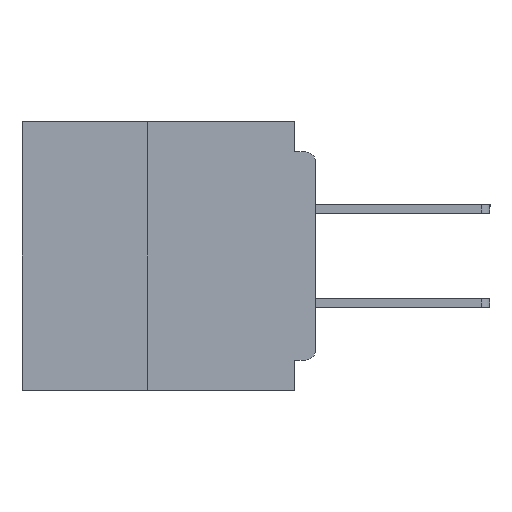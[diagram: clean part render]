
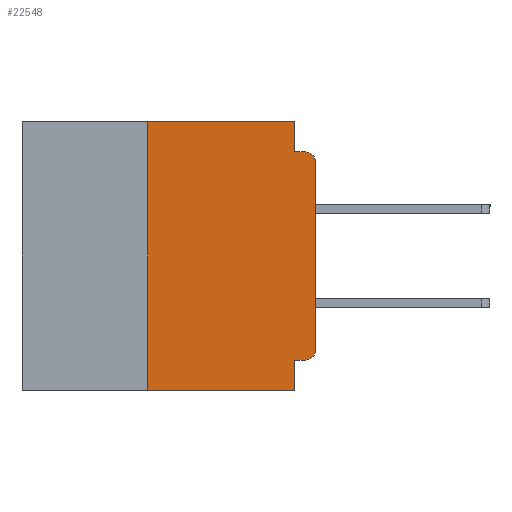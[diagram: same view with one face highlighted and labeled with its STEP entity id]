
A CAD part, left-side view. The second image highlights one B-rep face of the part: STEP entity #22548.
In plain terms, the highlighted planar face has unit normal (-1, 0, 0).
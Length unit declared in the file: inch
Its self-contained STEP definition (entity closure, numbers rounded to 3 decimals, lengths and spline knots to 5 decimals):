
#13 = CARTESIAN_POINT ( 'NONE',  ( 0., 0.25, -0.4 ) ) ;
#24 = VECTOR ( 'NONE', #770, 39.37008 ) ;
#57 = ORIENTED_EDGE ( 'NONE', *, *, #15353, .F. ) ;
#374 = VECTOR ( 'NONE', #3864, 39.37008 ) ;
#440 = EDGE_CURVE ( 'NONE', #1643, #30247, #30503, .T. ) ;
#537 = CARTESIAN_POINT ( 'NONE',  ( 0., 0.031, -0.355 ) ) ;
#770 = DIRECTION ( 'NONE',  ( 0., 0., -1. ) ) ;
#933 = PLANE ( 'NONE',  #33483 ) ;
#1409 = VECTOR ( 'NONE', #37729, 39.37008 ) ;
#1643 = VERTEX_POINT ( 'NONE', #7829 ) ;
#1731 = DIRECTION ( 'NONE',  ( -1., 0., 0. ) ) ;
#3371 = ORIENTED_EDGE ( 'NONE', *, *, #20092, .T. ) ;
#3565 = VECTOR ( 'NONE', #8889, 39.37008 ) ;
#3864 = DIRECTION ( 'NONE',  ( 0., 1., 0. ) ) ;
#4212 = ORIENTED_EDGE ( 'NONE', *, *, #440, .T. ) ;
#4406 = DIRECTION ( 'NONE',  ( 1., 0., 0. ) ) ;
#4809 = CARTESIAN_POINT ( 'NONE',  ( 0., 0.015, -0.355 ) ) ;
#5507 = FACE_OUTER_BOUND ( 'NONE', #14350, .T. ) ;
#5531 = EDGE_CURVE ( 'NONE', #20510, #21831, #27587, .T. ) ;
#6619 = VECTOR ( 'NONE', #39755, 39.37008 ) ;
#7664 = CARTESIAN_POINT ( 'NONE',  ( 0., 0.031, -0.4 ) ) ;
#7829 = CARTESIAN_POINT ( 'NONE',  ( 0., 0., -0.34 ) ) ;
#8083 = CARTESIAN_POINT ( 'NONE',  ( 0., 0., 0. ) ) ;
#8889 = DIRECTION ( 'NONE',  ( 0., 0., 1. ) ) ;
#9488 = LINE ( 'NONE', #24096, #374 ) ;
#9663 = VECTOR ( 'NONE', #23730, 39.37008 ) ;
#9683 = CARTESIAN_POINT ( 'NONE',  ( 0., 0.031, -0.045 ) ) ;
#10319 = VECTOR ( 'NONE', #42695, 39.37008 ) ;
#11229 = CARTESIAN_POINT ( 'NONE',  ( 0., 0.25, -0.4 ) ) ;
#11348 = ORIENTED_EDGE ( 'NONE', *, *, #22163, .F. ) ;
#11787 = AXIS2_PLACEMENT_3D ( 'NONE', #33454, #13274, #36806 ) ;
#12502 = ORIENTED_EDGE ( 'NONE', *, *, #20429, .F. ) ;
#13088 = AXIS2_PLACEMENT_3D ( 'NONE', #22023, #1731, #25389 ) ;
#13131 = ORIENTED_EDGE ( 'NONE', *, *, #18380, .F. ) ;
#13274 = DIRECTION ( 'NONE',  ( -1., 0., 0. ) ) ;
#13644 = ORIENTED_EDGE ( 'NONE', *, *, #39653, .T. ) ;
#14350 = EDGE_LOOP ( 'NONE', ( #4212, #3371, #12502, #11348, #13131, #14463, #23778, #57, #21104, #13644 ) ) ;
#14413 = DIRECTION ( 'NONE',  ( 0., -1., 0. ) ) ;
#14463 = ORIENTED_EDGE ( 'NONE', *, *, #5531, .F. ) ;
#15353 = EDGE_CURVE ( 'NONE', #21858, #39246, #27051, .T. ) ;
#17313 = CARTESIAN_POINT ( 'NONE',  ( 0., 0.25, 0. ) ) ;
#17541 = CARTESIAN_POINT ( 'NONE',  ( 0., 0., -0.045 ) ) ;
#18213 = LINE ( 'NONE', #19193, #10319 ) ;
#18380 = EDGE_CURVE ( 'NONE', #21831, #26326, #36759, .T. ) ;
#19193 = CARTESIAN_POINT ( 'NONE',  ( 0., 0.031, 0. ) ) ;
#20092 = EDGE_CURVE ( 'NONE', #30247, #25281, #22117, .T. ) ;
#20429 = EDGE_CURVE ( 'NONE', #27389, #25281, #27346, .T. ) ;
#20510 = VERTEX_POINT ( 'NONE', #11229 ) ;
#20982 = VECTOR ( 'NONE', #14413, 39.37008 ) ;
#21104 = ORIENTED_EDGE ( 'NONE', *, *, #40461, .F. ) ;
#21466 = CARTESIAN_POINT ( 'NONE',  ( 0., 0., -0.06 ) ) ;
#21831 = VERTEX_POINT ( 'NONE', #17313 ) ;
#21858 = VERTEX_POINT ( 'NONE', #537 ) ;
#22023 = CARTESIAN_POINT ( 'NONE',  ( 0., 0.015, -0.06 ) ) ;
#22117 = CIRCLE ( 'NONE', #13088, 0.015 ) ;
#22163 = EDGE_CURVE ( 'NONE', #26326, #27389, #18213, .T. ) ;
#22548 = ADVANCED_FACE ( 'NONE', ( #5507 ), #933, .F. ) ;
#23253 = CIRCLE ( 'NONE', #11787, 0.015 ) ;
#23525 = LINE ( 'NONE', #26375, #6619 ) ;
#23730 = DIRECTION ( 'NONE',  ( 0., 0., 1. ) ) ;
#23778 = ORIENTED_EDGE ( 'NONE', *, *, #32765, .T. ) ;
#24096 = CARTESIAN_POINT ( 'NONE',  ( 0., 0., -0.355 ) ) ;
#25281 = VERTEX_POINT ( 'NONE', #35893 ) ;
#25389 = DIRECTION ( 'NONE',  ( 0., 0., -1. ) ) ;
#26326 = VERTEX_POINT ( 'NONE', #38028 ) ;
#26375 = CARTESIAN_POINT ( 'NONE',  ( 0., 0.437, -0.4 ) ) ;
#27051 = LINE ( 'NONE', #37854, #24 ) ;
#27346 = LINE ( 'NONE', #17541, #1409 ) ;
#27389 = VERTEX_POINT ( 'NONE', #9683 ) ;
#27587 = LINE ( 'NONE', #13, #9663 ) ;
#27986 = DIRECTION ( 'NONE',  ( 0., 0., -1. ) ) ;
#29663 = VERTEX_POINT ( 'NONE', #4809 ) ;
#30247 = VERTEX_POINT ( 'NONE', #21466 ) ;
#30503 = LINE ( 'NONE', #8083, #3565 ) ;
#32765 = EDGE_CURVE ( 'NONE', #20510, #39246, #23525, .T. ) ;
#33454 = CARTESIAN_POINT ( 'NONE',  ( 0., 0.015, -0.34 ) ) ;
#33483 = AXIS2_PLACEMENT_3D ( 'NONE', #38010, #4406, #27986 ) ;
#35893 = CARTESIAN_POINT ( 'NONE',  ( 0., 0.015, -0.045 ) ) ;
#36759 = LINE ( 'NONE', #37959, #20982 ) ;
#36806 = DIRECTION ( 'NONE',  ( 0., 0., -1. ) ) ;
#37729 = DIRECTION ( 'NONE',  ( 0., -1., 0. ) ) ;
#37854 = CARTESIAN_POINT ( 'NONE',  ( 0., 0.031, -0.4 ) ) ;
#37959 = CARTESIAN_POINT ( 'NONE',  ( 0., 0.437, 0. ) ) ;
#38010 = CARTESIAN_POINT ( 'NONE',  ( 0., 0.437, 0. ) ) ;
#38028 = CARTESIAN_POINT ( 'NONE',  ( 0., 0.031, 0. ) ) ;
#39246 = VERTEX_POINT ( 'NONE', #7664 ) ;
#39653 = EDGE_CURVE ( 'NONE', #29663, #1643, #23253, .T. ) ;
#39755 = DIRECTION ( 'NONE',  ( 0., -1., 0. ) ) ;
#40461 = EDGE_CURVE ( 'NONE', #29663, #21858, #9488, .T. ) ;
#42695 = DIRECTION ( 'NONE',  ( 0., 0., -1. ) ) ;
